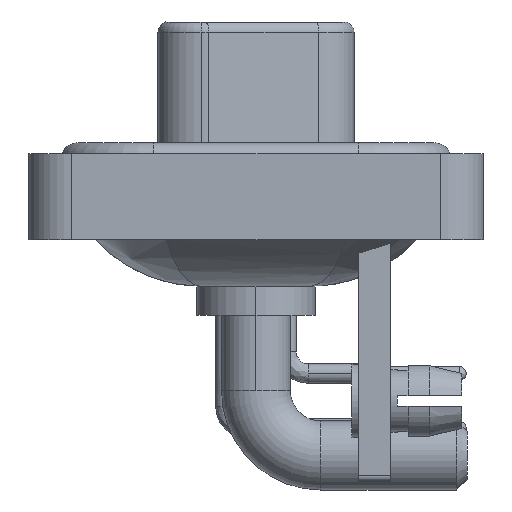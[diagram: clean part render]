
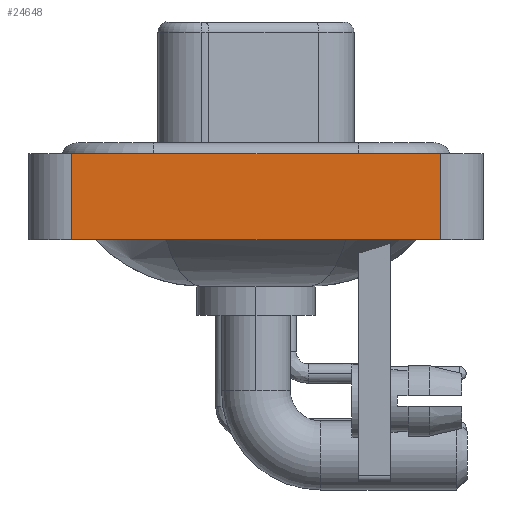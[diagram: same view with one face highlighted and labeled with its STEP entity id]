
A CAD part, left-side view. The second image highlights one B-rep face of the part: STEP entity #24648.
In plain terms, the highlighted planar face has unit normal (-1, 0, 0).
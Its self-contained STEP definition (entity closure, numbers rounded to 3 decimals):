
#1759 = CARTESIAN_POINT ( 'NONE',  ( -7.3, -8.55, -3.6 ) ) ;
#1880 = DIRECTION ( 'NONE',  ( 0., 0., 1. ) ) ;
#2047 = DIRECTION ( 'NONE',  ( -1., 0., 0. ) ) ;
#2158 = DIRECTION ( 'NONE',  ( 0., 0., 1. ) ) ;
#2285 = CARTESIAN_POINT ( 'NONE',  ( -7.3, 8.55, -3.6 ) ) ;
#2521 = EDGE_CURVE ( 'NONE', #10146, #7409, #3917, .T. ) ;
#2522 = AXIS2_PLACEMENT_3D ( 'NONE', #3664, #2047, #8277 ) ;
#3664 = CARTESIAN_POINT ( 'NONE',  ( -7.3, -8.55, -3.6 ) ) ;
#3761 = ORIENTED_EDGE ( 'NONE', *, *, #6983, .F. ) ;
#3917 = LINE ( 'NONE', #6457, #20347 ) ;
#5048 = DIRECTION ( 'NONE',  ( 0., -1., 0. ) ) ;
#6457 = CARTESIAN_POINT ( 'NONE',  ( -7.3, 8.55, -3.6 ) ) ;
#6983 = EDGE_CURVE ( 'NONE', #7409, #17689, #8224, .T. ) ;
#7409 = VERTEX_POINT ( 'NONE', #18280 ) ;
#8224 = LINE ( 'NONE', #16121, #11099 ) ;
#8239 = ORIENTED_EDGE ( 'NONE', *, *, #13840, .T. ) ;
#8277 = DIRECTION ( 'NONE',  ( 0., 0., 1. ) ) ;
#8355 = DIRECTION ( 'NONE',  ( 0., -1., 0. ) ) ;
#10146 = VERTEX_POINT ( 'NONE', #2285 ) ;
#10779 = CARTESIAN_POINT ( 'NONE',  ( -7.3, -8.55, -3.6 ) ) ;
#10965 = LINE ( 'NONE', #18885, #25909 ) ;
#11099 = VECTOR ( 'NONE', #8355, 1000. ) ;
#11310 = VERTEX_POINT ( 'NONE', #1759 ) ;
#11315 = LINE ( 'NONE', #10779, #18329 ) ;
#13840 = EDGE_CURVE ( 'NONE', #11310, #17689, #10965, .T. ) ;
#14010 = PLANE ( 'NONE',  #2522 ) ;
#16004 = ORIENTED_EDGE ( 'NONE', *, *, #2521, .F. ) ;
#16121 = CARTESIAN_POINT ( 'NONE',  ( -7.3, -8.55, 0.4 ) ) ;
#17689 = VERTEX_POINT ( 'NONE', #18506 ) ;
#18280 = CARTESIAN_POINT ( 'NONE',  ( -7.3, 8.55, 0.4 ) ) ;
#18329 = VECTOR ( 'NONE', #5048, 1000. ) ;
#18506 = CARTESIAN_POINT ( 'NONE',  ( -7.3, -8.55, 0.4 ) ) ;
#18885 = CARTESIAN_POINT ( 'NONE',  ( -7.3, -8.55, -3.6 ) ) ;
#19457 = EDGE_CURVE ( 'NONE', #10146, #11310, #11315, .T. ) ;
#20347 = VECTOR ( 'NONE', #1880, 1000. ) ;
#24379 = FACE_OUTER_BOUND ( 'NONE', #26668, .T. ) ;
#24648 = ADVANCED_FACE ( 'NONE', ( #24379 ), #14010, .T. ) ;
#25909 = VECTOR ( 'NONE', #2158, 1000. ) ;
#26668 = EDGE_LOOP ( 'NONE', ( #8239, #3761, #16004, #26918 ) ) ;
#26918 = ORIENTED_EDGE ( 'NONE', *, *, #19457, .T. ) ;
